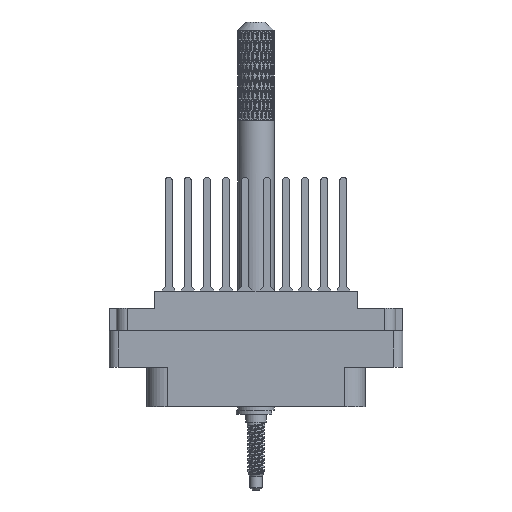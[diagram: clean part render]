
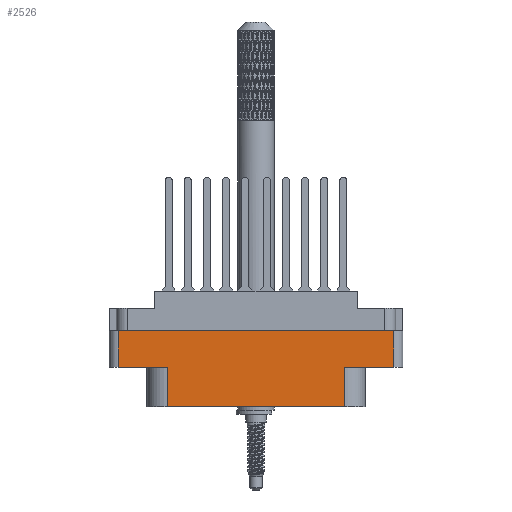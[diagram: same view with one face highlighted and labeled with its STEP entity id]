
A CAD part, front view. The second image highlights one B-rep face of the part: STEP entity #2526.
In plain terms, the highlighted planar face has unit normal (0, -1, 0).
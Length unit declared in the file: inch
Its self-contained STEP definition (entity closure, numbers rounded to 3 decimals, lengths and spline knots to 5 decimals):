
#1747 = VERTEX_POINT ( 'NONE', #13404 ) ;
#2526 = ADVANCED_FACE ( 'NONE', ( #2826 ), #29022, .T. ) ;
#2826 = FACE_OUTER_BOUND ( 'NONE', #41676, .T. ) ;
#5111 = EDGE_CURVE ( 'NONE', #60807, #31386, #12526, .T. ) ;
#6230 = LINE ( 'NONE', #92564, #18798 ) ;
#6244 = VERTEX_POINT ( 'NONE', #54818 ) ;
#6881 = CARTESIAN_POINT ( 'NONE',  ( 0., -0.438, -0.268 ) ) ;
#7091 = VECTOR ( 'NONE', #29584, 39.37008 ) ;
#11914 = CARTESIAN_POINT ( 'NONE',  ( 0., -0.438, -0.52 ) ) ;
#11931 = CARTESIAN_POINT ( 'NONE',  ( -0.938, -0.438, -0.52 ) ) ;
#12502 = EDGE_CURVE ( 'NONE', #62433, #6244, #74872, .T. ) ;
#12526 = LINE ( 'NONE', #6881, #73700 ) ;
#12639 = DIRECTION ( 'NONE',  ( 0., -1., 0. ) ) ;
#13328 = LINE ( 'NONE', #36888, #7091 ) ;
#13404 = CARTESIAN_POINT ( 'NONE',  ( 0.604, -0.438, -0.52 ) ) ;
#15340 = ORIENTED_EDGE ( 'NONE', *, *, #57272, .T. ) ;
#16468 = VERTEX_POINT ( 'NONE', #97781 ) ;
#18302 = VECTOR ( 'NONE', #86927, 39.37008 ) ;
#18480 = DIRECTION ( 'NONE',  ( 0., 0., 1. ) ) ;
#18505 = LINE ( 'NONE', #53023, #44685 ) ;
#18798 = VECTOR ( 'NONE', #76834, 39.37008 ) ;
#19898 = CARTESIAN_POINT ( 'NONE',  ( -0.938, -0.438, -0.268 ) ) ;
#28491 = ORIENTED_EDGE ( 'NONE', *, *, #56157, .T. ) ;
#29022 = PLANE ( 'NONE',  #70682 ) ;
#29488 = ORIENTED_EDGE ( 'NONE', *, *, #87298, .T. ) ;
#29584 = DIRECTION ( 'NONE',  ( 0., 0., 1. ) ) ;
#30218 = ORIENTED_EDGE ( 'NONE', *, *, #5111, .F. ) ;
#31386 = VERTEX_POINT ( 'NONE', #68221 ) ;
#32061 = CARTESIAN_POINT ( 'NONE',  ( -0.938, -0.438, -0.789 ) ) ;
#32623 = ORIENTED_EDGE ( 'NONE', *, *, #66960, .T. ) ;
#32864 = VERTEX_POINT ( 'NONE', #87794 ) ;
#36888 = CARTESIAN_POINT ( 'NONE',  ( 0.938, -0.438, -0.789 ) ) ;
#39386 = EDGE_CURVE ( 'NONE', #32864, #1747, #6230, .T. ) ;
#40822 = LINE ( 'NONE', #32061, #18302 ) ;
#41676 = EDGE_LOOP ( 'NONE', ( #30218, #15340, #49894, #49241, #28491, #29488, #52005, #32623 ) ) ;
#42124 = VERTEX_POINT ( 'NONE', #11931 ) ;
#44685 = VECTOR ( 'NONE', #94231, 39.37008 ) ;
#46213 = VECTOR ( 'NONE', #18480, 39.37008 ) ;
#49241 = ORIENTED_EDGE ( 'NONE', *, *, #12502, .T. ) ;
#49503 = EDGE_CURVE ( 'NONE', #42124, #62433, #57495, .T. ) ;
#49894 = ORIENTED_EDGE ( 'NONE', *, *, #49503, .T. ) ;
#52005 = ORIENTED_EDGE ( 'NONE', *, *, #39386, .F. ) ;
#53023 = CARTESIAN_POINT ( 'NONE',  ( -1., -0.438, -0.789 ) ) ;
#54818 = CARTESIAN_POINT ( 'NONE',  ( -0.604, -0.438, -0.789 ) ) ;
#56157 = EDGE_CURVE ( 'NONE', #6244, #16468, #18505, .T. ) ;
#57272 = EDGE_CURVE ( 'NONE', #60807, #42124, #40822, .T. ) ;
#57495 = LINE ( 'NONE', #11914, #58707 ) ;
#58707 = VECTOR ( 'NONE', #84170, 39.37008 ) ;
#60807 = VERTEX_POINT ( 'NONE', #19898 ) ;
#61144 = DIRECTION ( 'NONE',  ( 0., 0., -1. ) ) ;
#62121 = DIRECTION ( 'NONE',  ( 1., 0., 0. ) ) ;
#62433 = VERTEX_POINT ( 'NONE', #62673 ) ;
#62673 = CARTESIAN_POINT ( 'NONE',  ( -0.604, -0.438, -0.52 ) ) ;
#66860 = DIRECTION ( 'NONE',  ( 0., 0., -1. ) ) ;
#66960 = EDGE_CURVE ( 'NONE', #32864, #31386, #13328, .T. ) ;
#67522 = LINE ( 'NONE', #91081, #46213 ) ;
#68221 = CARTESIAN_POINT ( 'NONE',  ( 0.938, -0.438, -0.268 ) ) ;
#70682 = AXIS2_PLACEMENT_3D ( 'NONE', #84208, #12639, #61144 ) ;
#72386 = VECTOR ( 'NONE', #66860, 39.37008 ) ;
#73700 = VECTOR ( 'NONE', #62121, 39.37008 ) ;
#74872 = LINE ( 'NONE', #91987, #72386 ) ;
#76834 = DIRECTION ( 'NONE',  ( -1., 0., 0. ) ) ;
#84170 = DIRECTION ( 'NONE',  ( 1., 0., 0. ) ) ;
#84208 = CARTESIAN_POINT ( 'NONE',  ( -1., -0.438, -0.789 ) ) ;
#86927 = DIRECTION ( 'NONE',  ( 0., 0., -1. ) ) ;
#87298 = EDGE_CURVE ( 'NONE', #16468, #1747, #67522, .T. ) ;
#87794 = CARTESIAN_POINT ( 'NONE',  ( 0.938, -0.438, -0.52 ) ) ;
#91081 = CARTESIAN_POINT ( 'NONE',  ( 0.604, -0.438, -0.52 ) ) ;
#91987 = CARTESIAN_POINT ( 'NONE',  ( -0.604, -0.438, -0.789 ) ) ;
#92564 = CARTESIAN_POINT ( 'NONE',  ( 0., -0.438, -0.52 ) ) ;
#94231 = DIRECTION ( 'NONE',  ( 1., 0., 0. ) ) ;
#97781 = CARTESIAN_POINT ( 'NONE',  ( 0.604, -0.438, -0.789 ) ) ;
